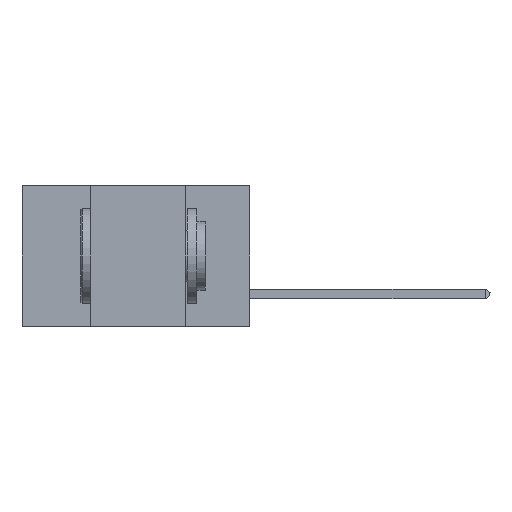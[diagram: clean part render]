
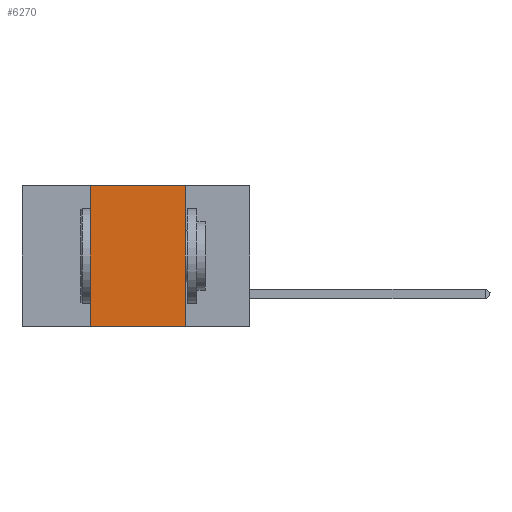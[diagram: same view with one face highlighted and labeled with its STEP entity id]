
A CAD part, left-side view. The second image highlights one B-rep face of the part: STEP entity #6270.
In plain terms, the highlighted planar face has unit normal (-1, 0, 0).
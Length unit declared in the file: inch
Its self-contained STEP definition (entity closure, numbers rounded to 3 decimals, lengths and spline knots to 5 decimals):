
#1520 = VECTOR ( 'NONE', #19326, 39.37008 ) ;
#1884 = EDGE_CURVE ( 'NONE', #9129, #24412, #3597, .T. ) ;
#2885 = PLANE ( 'NONE',  #14645 ) ;
#2987 = ORIENTED_EDGE ( 'NONE', *, *, #24787, .F. ) ;
#3249 = CARTESIAN_POINT ( 'NONE',  ( 0., 0.42, 0. ) ) ;
#3504 = EDGE_CURVE ( 'NONE', #12456, #9129, #23677, .T. ) ;
#3597 = LINE ( 'NONE', #10101, #5492 ) ;
#3905 = FACE_OUTER_BOUND ( 'NONE', #17496, .T. ) ;
#3911 = CARTESIAN_POINT ( 'NONE',  ( 0., 0.42, 0. ) ) ;
#4036 = DIRECTION ( 'NONE',  ( 0., 0., -1. ) ) ;
#5079 = DIRECTION ( 'NONE',  ( 1., 0., 0. ) ) ;
#5469 = CARTESIAN_POINT ( 'NONE',  ( 0., 0.42, -0.37 ) ) ;
#5492 = VECTOR ( 'NONE', #4036, 39.37008 ) ;
#6020 = VECTOR ( 'NONE', #9727, 39.37008 ) ;
#6270 = ADVANCED_FACE ( 'NONE', ( #3905 ), #2885, .F. ) ;
#8309 = LINE ( 'NONE', #3911, #10472 ) ;
#9129 = VERTEX_POINT ( 'NONE', #11378 ) ;
#9727 = DIRECTION ( 'NONE',  ( 0., -1., 0. ) ) ;
#10055 = CARTESIAN_POINT ( 'NONE',  ( 0., 0.6, 0. ) ) ;
#10101 = CARTESIAN_POINT ( 'NONE',  ( 0., 0.17, 0. ) ) ;
#10472 = VECTOR ( 'NONE', #21904, 39.37008 ) ;
#11378 = CARTESIAN_POINT ( 'NONE',  ( 0., 0.17, 0. ) ) ;
#12456 = VERTEX_POINT ( 'NONE', #3249 ) ;
#14317 = VERTEX_POINT ( 'NONE', #5469 ) ;
#14645 = AXIS2_PLACEMENT_3D ( 'NONE', #16976, #5079, #18985 ) ;
#15895 = ORIENTED_EDGE ( 'NONE', *, *, #24586, .T. ) ;
#16663 = ORIENTED_EDGE ( 'NONE', *, *, #3504, .F. ) ;
#16976 = CARTESIAN_POINT ( 'NONE',  ( 0., 0.6, 0. ) ) ;
#17496 = EDGE_LOOP ( 'NONE', ( #20852, #16663, #2987, #15895 ) ) ;
#18813 = CARTESIAN_POINT ( 'NONE',  ( 0., 0.6, -0.37 ) ) ;
#18985 = DIRECTION ( 'NONE',  ( 0., 0., -1. ) ) ;
#19326 = DIRECTION ( 'NONE',  ( 0., -1., 0. ) ) ;
#20852 = ORIENTED_EDGE ( 'NONE', *, *, #1884, .F. ) ;
#21422 = LINE ( 'NONE', #18813, #1520 ) ;
#21904 = DIRECTION ( 'NONE',  ( 0., 0., 1. ) ) ;
#23677 = LINE ( 'NONE', #10055, #6020 ) ;
#24276 = CARTESIAN_POINT ( 'NONE',  ( 0., 0.17, -0.37 ) ) ;
#24412 = VERTEX_POINT ( 'NONE', #24276 ) ;
#24586 = EDGE_CURVE ( 'NONE', #14317, #24412, #21422, .T. ) ;
#24787 = EDGE_CURVE ( 'NONE', #14317, #12456, #8309, .T. ) ;
